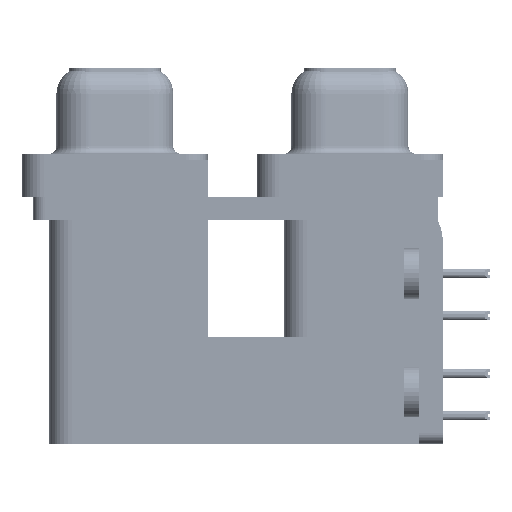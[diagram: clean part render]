
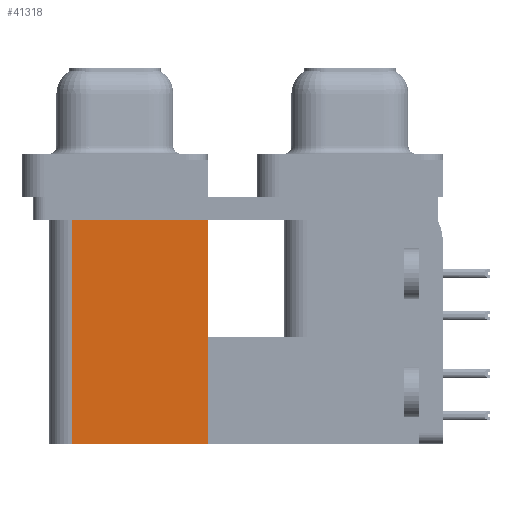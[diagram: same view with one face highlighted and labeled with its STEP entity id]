
A CAD part, left-side view. The second image highlights one B-rep face of the part: STEP entity #41318.
In plain terms, the highlighted planar face has unit normal (-1, 0, 0).
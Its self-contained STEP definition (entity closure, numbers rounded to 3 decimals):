
#909 = VERTEX_POINT ( 'NONE', #39101 ) ;
#3854 = CARTESIAN_POINT ( 'NONE',  ( 3.7, 18.8, -19.2 ) ) ;
#7006 = LINE ( 'NONE', #51562, #40682 ) ;
#10893 = VERTEX_POINT ( 'NONE', #33414 ) ;
#12722 = DIRECTION ( 'NONE',  ( 0., 1., 0. ) ) ;
#14621 = DIRECTION ( 'NONE',  ( 0., 0., 1. ) ) ;
#14658 = VECTOR ( 'NONE', #14621, 1000. ) ;
#14870 = EDGE_CURVE ( 'NONE', #909, #34914, #51794, .T. ) ;
#16546 = DIRECTION ( 'NONE',  ( 0., 0., 1. ) ) ;
#17593 = CARTESIAN_POINT ( 'NONE',  ( 3.7, 9.6, -2.5 ) ) ;
#17809 = CARTESIAN_POINT ( 'NONE',  ( 3.7, 9.6, -19.2 ) ) ;
#18150 = CARTESIAN_POINT ( 'NONE',  ( 3.7, 9.6, -19.2 ) ) ;
#21232 = ORIENTED_EDGE ( 'NONE', *, *, #14870, .F. ) ;
#21974 = ORIENTED_EDGE ( 'NONE', *, *, #54932, .T. ) ;
#22195 = CARTESIAN_POINT ( 'NONE',  ( 3.7, 9.6, -19.2 ) ) ;
#23224 = LINE ( 'NONE', #18150, #14658 ) ;
#27982 = PLANE ( 'NONE',  #57015 ) ;
#28547 = EDGE_LOOP ( 'NONE', ( #50288, #44114, #21232, #21974 ) ) ;
#28612 = DIRECTION ( 'NONE',  ( 1., 0., 0. ) ) ;
#32743 = FACE_OUTER_BOUND ( 'NONE', #28547, .T. ) ;
#33414 = CARTESIAN_POINT ( 'NONE',  ( 3.7, 18.8, -2.5 ) ) ;
#34914 = VERTEX_POINT ( 'NONE', #3854 ) ;
#36569 = EDGE_CURVE ( 'NONE', #34914, #10893, #60172, .T. ) ;
#39101 = CARTESIAN_POINT ( 'NONE',  ( 3.7, 9.6, -19.2 ) ) ;
#40682 = VECTOR ( 'NONE', #12722, 1000. ) ;
#41079 = EDGE_CURVE ( 'NONE', #50002, #10893, #7006, .T. ) ;
#41318 = ADVANCED_FACE ( 'NONE', ( #32743 ), #27982, .F. ) ;
#44114 = ORIENTED_EDGE ( 'NONE', *, *, #36569, .F. ) ;
#50002 = VERTEX_POINT ( 'NONE', #17593 ) ;
#50288 = ORIENTED_EDGE ( 'NONE', *, *, #41079, .T. ) ;
#51562 = CARTESIAN_POINT ( 'NONE',  ( 3.7, 9.6, -2.5 ) ) ;
#51794 = LINE ( 'NONE', #22195, #54931 ) ;
#52500 = DIRECTION ( 'NONE',  ( 0., 1., 0. ) ) ;
#54931 = VECTOR ( 'NONE', #56258, 1000. ) ;
#54932 = EDGE_CURVE ( 'NONE', #909, #50002, #23224, .T. ) ;
#55392 = CARTESIAN_POINT ( 'NONE',  ( 3.7, 18.8, -19.2 ) ) ;
#56258 = DIRECTION ( 'NONE',  ( 0., 1., 0. ) ) ;
#57015 = AXIS2_PLACEMENT_3D ( 'NONE', #17809, #28612, #52500 ) ;
#60172 = LINE ( 'NONE', #55392, #61896 ) ;
#61896 = VECTOR ( 'NONE', #16546, 1000. ) ;
